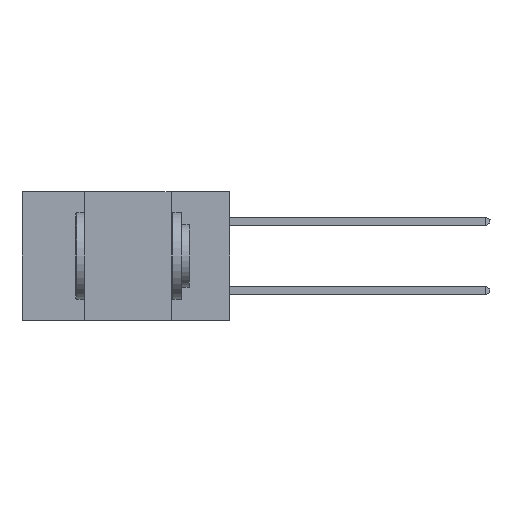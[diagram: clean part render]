
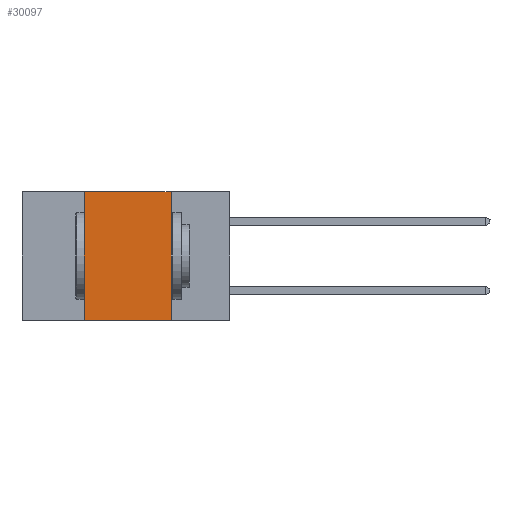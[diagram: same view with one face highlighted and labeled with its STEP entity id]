
A CAD part, left-side view. The second image highlights one B-rep face of the part: STEP entity #30097.
In plain terms, the highlighted planar face has unit normal (-1, 0, 0).
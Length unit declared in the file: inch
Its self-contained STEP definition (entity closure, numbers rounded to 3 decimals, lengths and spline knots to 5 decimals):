
#1203 = CARTESIAN_POINT ( 'NONE',  ( 0., 0.42, 0. ) ) ;
#1770 = DIRECTION ( 'NONE',  ( 0., -1., 0. ) ) ;
#2339 = DIRECTION ( 'NONE',  ( 0., -1., 0. ) ) ;
#2372 = VECTOR ( 'NONE', #1770, 39.37008 ) ;
#2591 = VERTEX_POINT ( 'NONE', #20665 ) ;
#5130 = VECTOR ( 'NONE', #29651, 39.37008 ) ;
#6010 = AXIS2_PLACEMENT_3D ( 'NONE', #21791, #24186, #9898 ) ;
#8425 = CARTESIAN_POINT ( 'NONE',  ( 0., 0.17, 0. ) ) ;
#8470 = CARTESIAN_POINT ( 'NONE',  ( 0., 0.42, 0. ) ) ;
#8704 = LINE ( 'NONE', #1203, #11676 ) ;
#8908 = EDGE_CURVE ( 'NONE', #16229, #17715, #8704, .T. ) ;
#9337 = ORIENTED_EDGE ( 'NONE', *, *, #22511, .F. ) ;
#9449 = LINE ( 'NONE', #15644, #2372 ) ;
#9898 = DIRECTION ( 'NONE',  ( 0., 0., -1. ) ) ;
#11218 = FACE_OUTER_BOUND ( 'NONE', #30647, .T. ) ;
#11676 = VECTOR ( 'NONE', #24743, 39.37008 ) ;
#13053 = CARTESIAN_POINT ( 'NONE',  ( 0., 0.42, -0.37 ) ) ;
#15578 = LINE ( 'NONE', #8425, #5130 ) ;
#15644 = CARTESIAN_POINT ( 'NONE',  ( 0., 0.6, -0.37 ) ) ;
#16229 = VERTEX_POINT ( 'NONE', #13053 ) ;
#16269 = ORIENTED_EDGE ( 'NONE', *, *, #8908, .F. ) ;
#17715 = VERTEX_POINT ( 'NONE', #8470 ) ;
#19372 = EDGE_CURVE ( 'NONE', #2591, #22893, #15578, .T. ) ;
#19452 = ORIENTED_EDGE ( 'NONE', *, *, #19372, .F. ) ;
#20665 = CARTESIAN_POINT ( 'NONE',  ( 0., 0.17, 0. ) ) ;
#20907 = CARTESIAN_POINT ( 'NONE',  ( 0., 0.6, 0. ) ) ;
#21606 = EDGE_CURVE ( 'NONE', #16229, #22893, #9449, .T. ) ;
#21791 = CARTESIAN_POINT ( 'NONE',  ( 0., 0.6, 0. ) ) ;
#22030 = LINE ( 'NONE', #20907, #26547 ) ;
#22187 = PLANE ( 'NONE',  #6010 ) ;
#22511 = EDGE_CURVE ( 'NONE', #17715, #2591, #22030, .T. ) ;
#22893 = VERTEX_POINT ( 'NONE', #25134 ) ;
#24186 = DIRECTION ( 'NONE',  ( 1., 0., 0. ) ) ;
#24237 = ORIENTED_EDGE ( 'NONE', *, *, #21606, .T. ) ;
#24743 = DIRECTION ( 'NONE',  ( 0., 0., 1. ) ) ;
#25134 = CARTESIAN_POINT ( 'NONE',  ( 0., 0.17, -0.37 ) ) ;
#26547 = VECTOR ( 'NONE', #2339, 39.37008 ) ;
#29651 = DIRECTION ( 'NONE',  ( 0., 0., -1. ) ) ;
#30097 = ADVANCED_FACE ( 'NONE', ( #11218 ), #22187, .F. ) ;
#30647 = EDGE_LOOP ( 'NONE', ( #19452, #9337, #16269, #24237 ) ) ;
